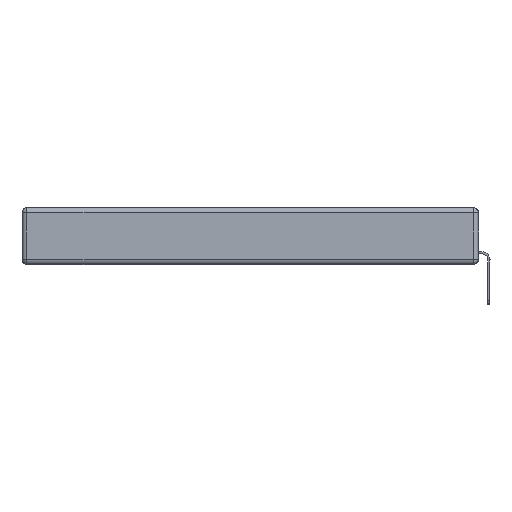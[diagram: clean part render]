
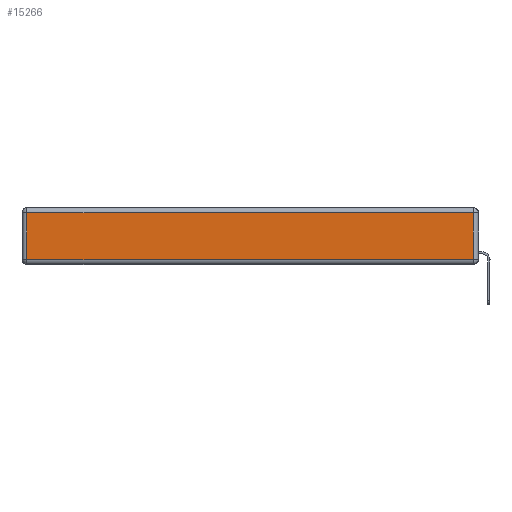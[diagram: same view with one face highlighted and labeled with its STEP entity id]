
A CAD part, left-side view. The second image highlights one B-rep face of the part: STEP entity #15266.
In plain terms, the highlighted planar face has unit normal (-1, 0, 0).
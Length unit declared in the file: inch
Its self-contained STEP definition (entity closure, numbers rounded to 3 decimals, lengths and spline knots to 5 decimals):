
#408 = EDGE_CURVE ( 'NONE', #7965, #1107, #7843, .T. ) ;
#1107 = VERTEX_POINT ( 'NONE', #16940 ) ;
#1184 = FACE_OUTER_BOUND ( 'NONE', #3567, .T. ) ;
#2056 = VECTOR ( 'NONE', #13350, 39.37008 ) ;
#2727 = ORIENTED_EDGE ( 'NONE', *, *, #13156, .T. ) ;
#3567 = EDGE_LOOP ( 'NONE', ( #17431, #16694, #11650, #2727 ) ) ;
#3806 = DIRECTION ( 'NONE',  ( 0., 0., -1. ) ) ;
#4158 = VERTEX_POINT ( 'NONE', #11629 ) ;
#5696 = DIRECTION ( 'NONE',  ( -1., 0., 0. ) ) ;
#7699 = CARTESIAN_POINT ( 'NONE',  ( 0., 0.03, -0.313 ) ) ;
#7843 = LINE ( 'NONE', #10342, #21165 ) ;
#7965 = VERTEX_POINT ( 'NONE', #7699 ) ;
#10151 = EDGE_CURVE ( 'NONE', #11242, #7965, #20039, .T. ) ;
#10342 = CARTESIAN_POINT ( 'NONE',  ( 0., 0.03, -0.343 ) ) ;
#10455 = LINE ( 'NONE', #18745, #14607 ) ;
#10643 = PLANE ( 'NONE',  #16008 ) ;
#11242 = VERTEX_POINT ( 'NONE', #16957 ) ;
#11629 = CARTESIAN_POINT ( 'NONE',  ( 0., 2.72, -0.03 ) ) ;
#11650 = ORIENTED_EDGE ( 'NONE', *, *, #14648, .T. ) ;
#12056 = CARTESIAN_POINT ( 'NONE',  ( 0., 0., -0.313 ) ) ;
#12261 = DIRECTION ( 'NONE',  ( 0., 0., 1. ) ) ;
#13156 = EDGE_CURVE ( 'NONE', #4158, #11242, #13601, .T. ) ;
#13350 = DIRECTION ( 'NONE',  ( 0., -1., 0. ) ) ;
#13601 = LINE ( 'NONE', #15543, #14559 ) ;
#14202 = CARTESIAN_POINT ( 'NONE',  ( 0., 0., -0.343 ) ) ;
#14559 = VECTOR ( 'NONE', #3806, 39.37008 ) ;
#14607 = VECTOR ( 'NONE', #18427, 39.37008 ) ;
#14648 = EDGE_CURVE ( 'NONE', #1107, #4158, #10455, .T. ) ;
#15266 = ADVANCED_FACE ( 'NONE', ( #1184 ), #10643, .T. ) ;
#15543 = CARTESIAN_POINT ( 'NONE',  ( 0., 2.72, -0.343 ) ) ;
#16008 = AXIS2_PLACEMENT_3D ( 'NONE', #14202, #5696, #12261 ) ;
#16694 = ORIENTED_EDGE ( 'NONE', *, *, #408, .T. ) ;
#16940 = CARTESIAN_POINT ( 'NONE',  ( 0., 0.03, -0.03 ) ) ;
#16957 = CARTESIAN_POINT ( 'NONE',  ( 0., 2.72, -0.313 ) ) ;
#17431 = ORIENTED_EDGE ( 'NONE', *, *, #10151, .T. ) ;
#17525 = DIRECTION ( 'NONE',  ( 0., 0., 1. ) ) ;
#18427 = DIRECTION ( 'NONE',  ( 0., 1., 0. ) ) ;
#18745 = CARTESIAN_POINT ( 'NONE',  ( 0., 2.75, -0.03 ) ) ;
#20039 = LINE ( 'NONE', #12056, #2056 ) ;
#21165 = VECTOR ( 'NONE', #17525, 39.37008 ) ;
